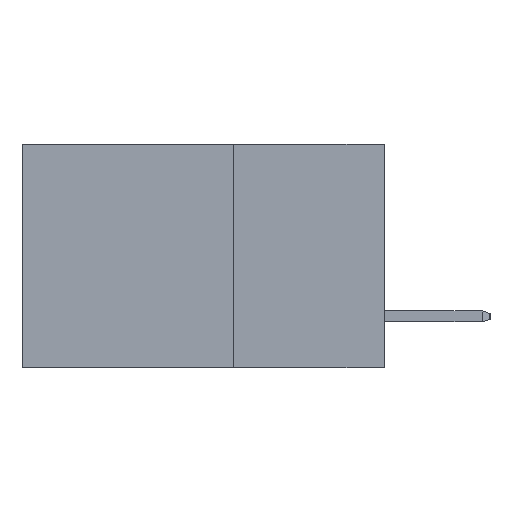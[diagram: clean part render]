
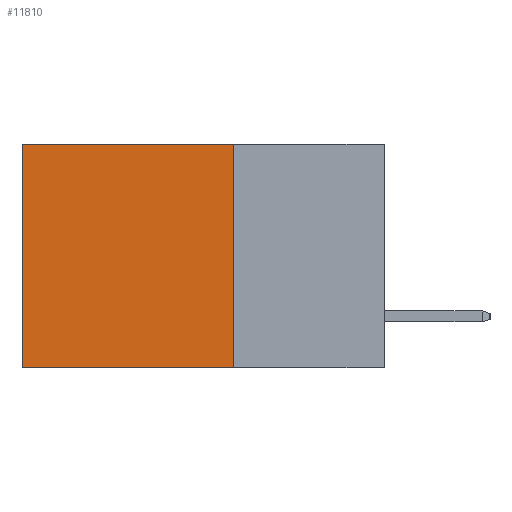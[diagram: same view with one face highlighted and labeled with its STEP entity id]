
A CAD part, left-side view. The second image highlights one B-rep face of the part: STEP entity #11810.
In plain terms, the highlighted planar face has unit normal (-1, 0, 0).
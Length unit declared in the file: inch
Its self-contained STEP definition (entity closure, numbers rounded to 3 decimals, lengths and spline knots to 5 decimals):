
#80 = VERTEX_POINT ( 'NONE', #203 ) ;
#203 = CARTESIAN_POINT ( 'NONE',  ( 0.2615, 0.6, -0.37 ) ) ;
#338 = VECTOR ( 'NONE', #6430, 39.37008 ) ;
#428 = DIRECTION ( 'NONE',  ( 1., 0., 0. ) ) ;
#1423 = VECTOR ( 'NONE', #6926, 39.37008 ) ;
#1605 = FACE_OUTER_BOUND ( 'NONE', #10184, .T. ) ;
#1948 = DIRECTION ( 'NONE',  ( 0., 1., 0. ) ) ;
#2260 = VERTEX_POINT ( 'NONE', #15645 ) ;
#2480 = VECTOR ( 'NONE', #8306, 39.37008 ) ;
#2630 = ORIENTED_EDGE ( 'NONE', *, *, #16244, .T. ) ;
#3312 = CARTESIAN_POINT ( 'NONE',  ( 0.2615, 0.6, 0. ) ) ;
#3449 = VERTEX_POINT ( 'NONE', #3312 ) ;
#3931 = LINE ( 'NONE', #15728, #338 ) ;
#4162 = CARTESIAN_POINT ( 'NONE',  ( 0.2615, 0.25, -0.37 ) ) ;
#4443 = PLANE ( 'NONE',  #11349 ) ;
#6114 = LINE ( 'NONE', #8244, #2480 ) ;
#6127 = LINE ( 'NONE', #8791, #15925 ) ;
#6430 = DIRECTION ( 'NONE',  ( 0., 1., 0. ) ) ;
#6926 = DIRECTION ( 'NONE',  ( 0., 0., -1. ) ) ;
#8040 = VERTEX_POINT ( 'NONE', #15778 ) ;
#8244 = CARTESIAN_POINT ( 'NONE',  ( 0.2615, 0.6, -0.37 ) ) ;
#8306 = DIRECTION ( 'NONE',  ( 0., 0., -1. ) ) ;
#8441 = ORIENTED_EDGE ( 'NONE', *, *, #11460, .F. ) ;
#8791 = CARTESIAN_POINT ( 'NONE',  ( 0.2615, 0.25, 0. ) ) ;
#9950 = EDGE_CURVE ( 'NONE', #2260, #3449, #6127, .T. ) ;
#10006 = DIRECTION ( 'NONE',  ( 0., 0., -1. ) ) ;
#10184 = EDGE_LOOP ( 'NONE', ( #2630, #8441, #13835, #10246 ) ) ;
#10246 = ORIENTED_EDGE ( 'NONE', *, *, #9950, .T. ) ;
#11147 = EDGE_CURVE ( 'NONE', #2260, #8040, #12226, .T. ) ;
#11349 = AXIS2_PLACEMENT_3D ( 'NONE', #15134, #428, #10006 ) ;
#11460 = EDGE_CURVE ( 'NONE', #8040, #80, #3931, .T. ) ;
#11810 = ADVANCED_FACE ( 'NONE', ( #1605 ), #4443, .F. ) ;
#12226 = LINE ( 'NONE', #4162, #1423 ) ;
#13835 = ORIENTED_EDGE ( 'NONE', *, *, #11147, .F. ) ;
#15134 = CARTESIAN_POINT ( 'NONE',  ( 0.2615, 0.25, -0.37 ) ) ;
#15645 = CARTESIAN_POINT ( 'NONE',  ( 0.2615, 0.25, 0. ) ) ;
#15728 = CARTESIAN_POINT ( 'NONE',  ( 0.2615, 0.25, -0.37 ) ) ;
#15778 = CARTESIAN_POINT ( 'NONE',  ( 0.2615, 0.25, -0.37 ) ) ;
#15925 = VECTOR ( 'NONE', #1948, 39.37008 ) ;
#16244 = EDGE_CURVE ( 'NONE', #3449, #80, #6114, .T. ) ;
